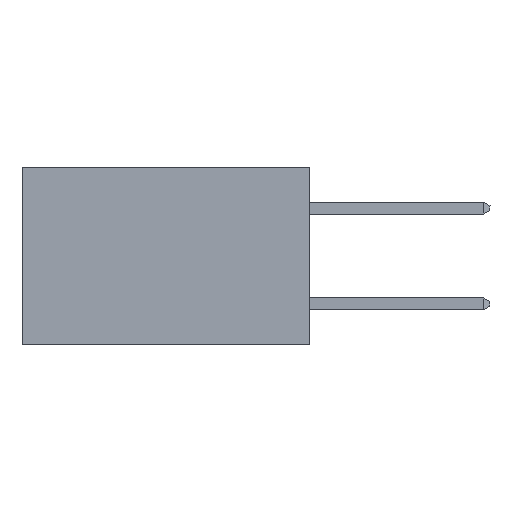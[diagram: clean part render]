
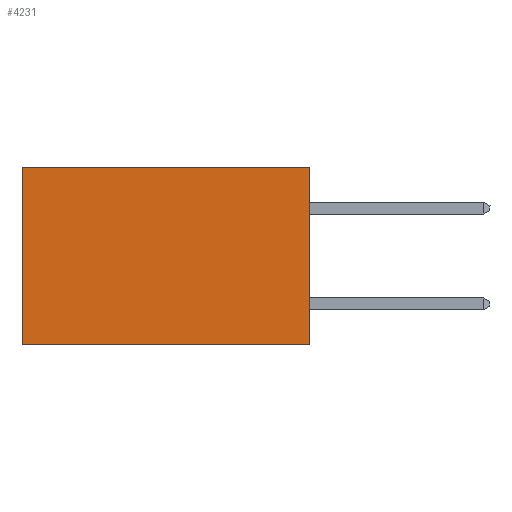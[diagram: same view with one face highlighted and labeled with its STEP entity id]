
A CAD part, left-side view. The second image highlights one B-rep face of the part: STEP entity #4231.
In plain terms, the highlighted planar face has unit normal (-1, 0, 0).
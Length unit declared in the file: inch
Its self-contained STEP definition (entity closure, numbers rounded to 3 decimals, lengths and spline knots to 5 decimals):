
#15 = EDGE_CURVE ( 'NONE', #6102, #4932, #6124, .T. ) ;
#491 = LINE ( 'NONE', #3013, #8485 ) ;
#732 = ORIENTED_EDGE ( 'NONE', *, *, #8566, .T. ) ;
#750 = VECTOR ( 'NONE', #11963, 39.37008 ) ;
#800 = CARTESIAN_POINT ( 'NONE',  ( 0.2875, 0., 0. ) ) ;
#1438 = ORIENTED_EDGE ( 'NONE', *, *, #15, .T. ) ;
#1668 = FACE_OUTER_BOUND ( 'NONE', #2785, .T. ) ;
#2021 = CARTESIAN_POINT ( 'NONE',  ( 0.2875, 0., -0.37 ) ) ;
#2057 = AXIS2_PLACEMENT_3D ( 'NONE', #12285, #12244, #12242 ) ;
#2206 = VECTOR ( 'NONE', #6148, 39.37008 ) ;
#2785 = EDGE_LOOP ( 'NONE', ( #732, #3057, #8775, #1438 ) ) ;
#3013 = CARTESIAN_POINT ( 'NONE',  ( 0.2875, 0.6, 0. ) ) ;
#3057 = ORIENTED_EDGE ( 'NONE', *, *, #12484, .F. ) ;
#3414 = VECTOR ( 'NONE', #3923, 39.37008 ) ;
#3923 = DIRECTION ( 'NONE',  ( 0., 1., 0. ) ) ;
#4051 = DIRECTION ( 'NONE',  ( 0., 0., -1. ) ) ;
#4231 = ADVANCED_FACE ( 'NONE', ( #1668 ), #12493, .F. ) ;
#4932 = VERTEX_POINT ( 'NONE', #5013 ) ;
#4946 = EDGE_CURVE ( 'NONE', #6102, #7628, #6302, .T. ) ;
#4968 = LINE ( 'NONE', #2021, #2206 ) ;
#5013 = CARTESIAN_POINT ( 'NONE',  ( 0.2875, 0.6, 0. ) ) ;
#5191 = CARTESIAN_POINT ( 'NONE',  ( 0.2875, 0.6, -0.37 ) ) ;
#6102 = VERTEX_POINT ( 'NONE', #12843 ) ;
#6124 = LINE ( 'NONE', #6856, #3414 ) ;
#6148 = DIRECTION ( 'NONE',  ( 0., 1., 0. ) ) ;
#6302 = LINE ( 'NONE', #800, #750 ) ;
#6856 = CARTESIAN_POINT ( 'NONE',  ( 0.2875, 0., 0. ) ) ;
#7628 = VERTEX_POINT ( 'NONE', #8338 ) ;
#8338 = CARTESIAN_POINT ( 'NONE',  ( 0.2875, 0., -0.37 ) ) ;
#8485 = VECTOR ( 'NONE', #4051, 39.37008 ) ;
#8566 = EDGE_CURVE ( 'NONE', #4932, #10612, #491, .T. ) ;
#8775 = ORIENTED_EDGE ( 'NONE', *, *, #4946, .F. ) ;
#10612 = VERTEX_POINT ( 'NONE', #5191 ) ;
#11963 = DIRECTION ( 'NONE',  ( 0., 0., -1. ) ) ;
#12242 = DIRECTION ( 'NONE',  ( 0., 0., -1. ) ) ;
#12244 = DIRECTION ( 'NONE',  ( 1., 0., 0. ) ) ;
#12285 = CARTESIAN_POINT ( 'NONE',  ( 0.2875, 0., 0. ) ) ;
#12484 = EDGE_CURVE ( 'NONE', #7628, #10612, #4968, .T. ) ;
#12493 = PLANE ( 'NONE',  #2057 ) ;
#12843 = CARTESIAN_POINT ( 'NONE',  ( 0.2875, 0., 0. ) ) ;
